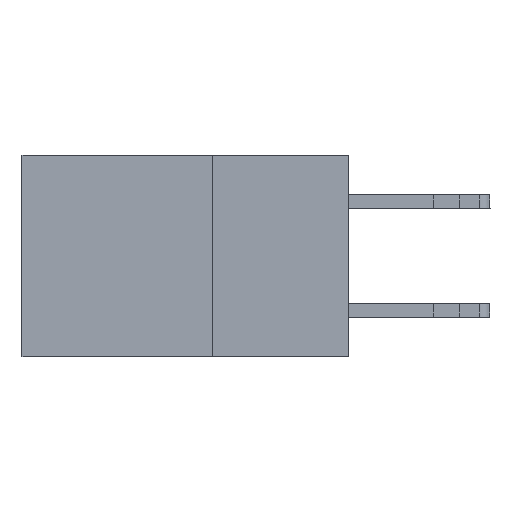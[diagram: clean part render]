
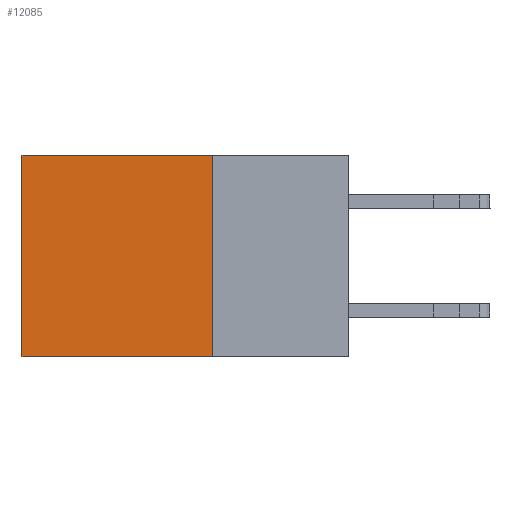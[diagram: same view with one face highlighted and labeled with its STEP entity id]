
A CAD part, left-side view. The second image highlights one B-rep face of the part: STEP entity #12085.
In plain terms, the highlighted planar face has unit normal (-1, 0, 0).
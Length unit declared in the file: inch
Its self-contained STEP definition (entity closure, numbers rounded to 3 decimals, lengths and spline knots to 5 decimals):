
#88 = CARTESIAN_POINT ( 'NONE',  ( 0.2615, 0.25, 0. ) ) ;
#182 = CARTESIAN_POINT ( 'NONE',  ( 0.2615, 0.6, -0.37 ) ) ;
#216 = VECTOR ( 'NONE', #11666, 39.37008 ) ;
#786 = CARTESIAN_POINT ( 'NONE',  ( 0.2615, 0.25, -0.37 ) ) ;
#992 = VERTEX_POINT ( 'NONE', #182 ) ;
#1596 = VECTOR ( 'NONE', #10507, 39.37008 ) ;
#2687 = CARTESIAN_POINT ( 'NONE',  ( 0.2615, 0.25, 0. ) ) ;
#2919 = EDGE_CURVE ( 'NONE', #9488, #992, #16452, .T. ) ;
#3243 = AXIS2_PLACEMENT_3D ( 'NONE', #19433, #19337, #9923 ) ;
#3351 = DIRECTION ( 'NONE',  ( 0., 0., -1. ) ) ;
#4939 = CARTESIAN_POINT ( 'NONE',  ( 0.2615, 0.6, 0. ) ) ;
#4985 = CARTESIAN_POINT ( 'NONE',  ( 0.2615, 0.25, -0.37 ) ) ;
#5157 = VECTOR ( 'NONE', #3351, 39.37008 ) ;
#7394 = ORIENTED_EDGE ( 'NONE', *, *, #2919, .F. ) ;
#7595 = DIRECTION ( 'NONE',  ( 0., 0., -1. ) ) ;
#7681 = EDGE_CURVE ( 'NONE', #13724, #10236, #16600, .T. ) ;
#7829 = EDGE_CURVE ( 'NONE', #13724, #9488, #11006, .T. ) ;
#8432 = EDGE_CURVE ( 'NONE', #10236, #992, #12726, .T. ) ;
#8454 = EDGE_LOOP ( 'NONE', ( #19380, #7394, #10069, #8706 ) ) ;
#8706 = ORIENTED_EDGE ( 'NONE', *, *, #7681, .T. ) ;
#9488 = VERTEX_POINT ( 'NONE', #786 ) ;
#9923 = DIRECTION ( 'NONE',  ( 0., 0., -1. ) ) ;
#10069 = ORIENTED_EDGE ( 'NONE', *, *, #7829, .F. ) ;
#10236 = VERTEX_POINT ( 'NONE', #4939 ) ;
#10507 = DIRECTION ( 'NONE',  ( 0., 1., 0. ) ) ;
#11006 = LINE ( 'NONE', #4985, #19214 ) ;
#11439 = FACE_OUTER_BOUND ( 'NONE', #8454, .T. ) ;
#11666 = DIRECTION ( 'NONE',  ( 0., 1., 0. ) ) ;
#12085 = ADVANCED_FACE ( 'NONE', ( #11439 ), #13300, .F. ) ;
#12726 = LINE ( 'NONE', #13962, #5157 ) ;
#13300 = PLANE ( 'NONE',  #3243 ) ;
#13724 = VERTEX_POINT ( 'NONE', #88 ) ;
#13962 = CARTESIAN_POINT ( 'NONE',  ( 0.2615, 0.6, -0.37 ) ) ;
#16160 = CARTESIAN_POINT ( 'NONE',  ( 0.2615, 0.25, -0.37 ) ) ;
#16452 = LINE ( 'NONE', #16160, #216 ) ;
#16600 = LINE ( 'NONE', #2687, #1596 ) ;
#19214 = VECTOR ( 'NONE', #7595, 39.37008 ) ;
#19337 = DIRECTION ( 'NONE',  ( 1., 0., 0. ) ) ;
#19380 = ORIENTED_EDGE ( 'NONE', *, *, #8432, .T. ) ;
#19433 = CARTESIAN_POINT ( 'NONE',  ( 0.2615, 0.25, -0.37 ) ) ;
